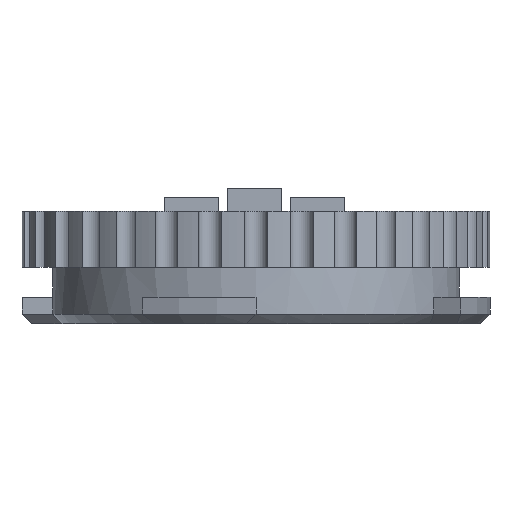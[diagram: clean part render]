
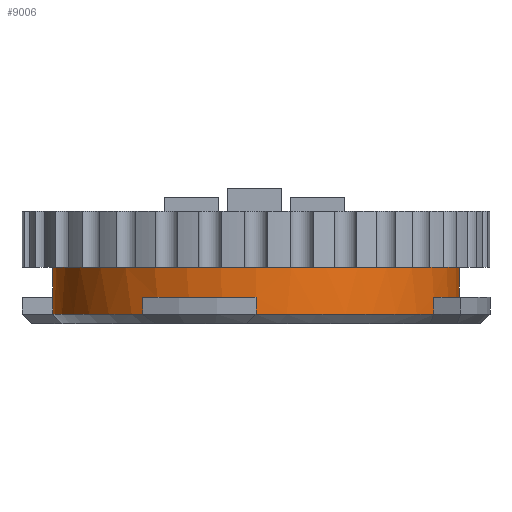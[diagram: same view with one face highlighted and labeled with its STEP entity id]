
A CAD part, front view. The second image highlights one B-rep face of the part: STEP entity #9006.
In plain terms, the highlighted cylindrical face has radius 13.787 mm (diameter 27.575 mm), a partial arc.
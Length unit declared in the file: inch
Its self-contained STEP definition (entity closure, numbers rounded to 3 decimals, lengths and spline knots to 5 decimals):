
#141 = EDGE_LOOP ( 'NONE', ( #9141, #763, #3634, #7107, #8365, #8469, #3518, #1365, #10371, #2251, #10949 ) ) ;
#189 = VECTOR ( 'NONE', #6156, 39.37008 ) ;
#298 = DIRECTION ( 'NONE',  ( 0., 0., 1. ) ) ;
#655 = LINE ( 'NONE', #5146, #10952 ) ;
#664 = DIRECTION ( 'NONE',  ( 1., 0., 0. ) ) ;
#696 = CARTESIAN_POINT ( 'NONE',  ( 0., 0., 0.02461 ) ) ;
#763 = ORIENTED_EDGE ( 'NONE', *, *, #4213, .F. ) ;
#806 = LINE ( 'NONE', #2953, #6941 ) ;
#832 = AXIS2_PLACEMENT_3D ( 'NONE', #9431, #8624, #664 ) ;
#866 = CARTESIAN_POINT ( 'NONE',  ( 0., -0.54281, 0.02461 ) ) ;
#1086 = DIRECTION ( 'NONE',  ( 0., 0., 1. ) ) ;
#1169 = CARTESIAN_POINT ( 'NONE',  ( 0.54281, 0., 0.15 ) ) ;
#1365 = ORIENTED_EDGE ( 'NONE', *, *, #7004, .T. ) ;
#1416 = DIRECTION ( 'NONE',  ( 1., 0., 0. ) ) ;
#1439 = CARTESIAN_POINT ( 'NONE',  ( 0., 0., 0.02461 ) ) ;
#1851 = VERTEX_POINT ( 'NONE', #9641 ) ;
#1888 = EDGE_CURVE ( 'NONE', #9745, #4321, #6204, .T. ) ;
#2251 = ORIENTED_EDGE ( 'NONE', *, *, #4976, .T. ) ;
#2330 = VERTEX_POINT ( 'NONE', #10304 ) ;
#2586 = CARTESIAN_POINT ( 'NONE',  ( 0., -0.54281, 0.15 ) ) ;
#2602 = DIRECTION ( 'NONE',  ( 0., 0., 1. ) ) ;
#2778 = CARTESIAN_POINT ( 'NONE',  ( -0.54281, 0., 0.07 ) ) ;
#2848 = DIRECTION ( 'NONE',  ( 0., 0., -1. ) ) ;
#2953 = CARTESIAN_POINT ( 'NONE',  ( -0.54281, 0., 0.15 ) ) ;
#2986 = EDGE_CURVE ( 'NONE', #6520, #3218, #8915, .T. ) ;
#3113 = EDGE_CURVE ( 'NONE', #11128, #8111, #8651, .T. ) ;
#3218 = VERTEX_POINT ( 'NONE', #11269 ) ;
#3281 = EDGE_CURVE ( 'NONE', #3218, #9745, #4130, .T. ) ;
#3293 = AXIS2_PLACEMENT_3D ( 'NONE', #7171, #298, #8107 ) ;
#3299 = CARTESIAN_POINT ( 'NONE',  ( 0.47476, -0.26316, 0.02461 ) ) ;
#3492 = VECTOR ( 'NONE', #2848, 39.37008 ) ;
#3518 = ORIENTED_EDGE ( 'NONE', *, *, #1888, .T. ) ;
#3634 = ORIENTED_EDGE ( 'NONE', *, *, #11001, .T. ) ;
#3752 = LINE ( 'NONE', #2586, #189 ) ;
#4087 = DIRECTION ( 'NONE',  ( 1., 0., 0. ) ) ;
#4117 = AXIS2_PLACEMENT_3D ( 'NONE', #9459, #7789, #7860 ) ;
#4130 = LINE ( 'NONE', #8966, #7940 ) ;
#4213 = EDGE_CURVE ( 'NONE', #1851, #10253, #10690, .T. ) ;
#4321 = VERTEX_POINT ( 'NONE', #9734 ) ;
#4491 = VECTOR ( 'NONE', #6603, 39.37008 ) ;
#4728 = LINE ( 'NONE', #1169, #3492 ) ;
#4976 = EDGE_CURVE ( 'NONE', #8111, #2330, #655, .T. ) ;
#5055 = VERTEX_POINT ( 'NONE', #2778 ) ;
#5146 = CARTESIAN_POINT ( 'NONE',  ( 0.47476, -0.26316, 0.15 ) ) ;
#5902 = DIRECTION ( 'NONE',  ( 0., 0., 1. ) ) ;
#6156 = DIRECTION ( 'NONE',  ( 0., 0., -1. ) ) ;
#6204 = CIRCLE ( 'NONE', #3293, 0.54281 ) ;
#6321 = FACE_OUTER_BOUND ( 'NONE', #141, .T. ) ;
#6477 = DIRECTION ( 'NONE',  ( 0., 0., -1. ) ) ;
#6520 = VERTEX_POINT ( 'NONE', #7871 ) ;
#6603 = DIRECTION ( 'NONE',  ( 0., 0., -1. ) ) ;
#6847 = DIRECTION ( 'NONE',  ( 1., 0., 0. ) ) ;
#6941 = VECTOR ( 'NONE', #6477, 39.37008 ) ;
#7004 = EDGE_CURVE ( 'NONE', #4321, #11128, #3752, .T. ) ;
#7107 = ORIENTED_EDGE ( 'NONE', *, *, #11328, .T. ) ;
#7136 = CYLINDRICAL_SURFACE ( 'NONE', #4117, 0.54281 ) ;
#7171 = CARTESIAN_POINT ( 'NONE',  ( 0., 0., 0.07 ) ) ;
#7276 = EDGE_CURVE ( 'NONE', #10253, #7650, #4728, .T. ) ;
#7650 = VERTEX_POINT ( 'NONE', #10517 ) ;
#7734 = DIRECTION ( 'NONE',  ( 0., 0., 1. ) ) ;
#7789 = DIRECTION ( 'NONE',  ( 0., 0., -1. ) ) ;
#7860 = DIRECTION ( 'NONE',  ( -1., 0., 0. ) ) ;
#7871 = CARTESIAN_POINT ( 'NONE',  ( -0.54281, 0., 0.02461 ) ) ;
#7940 = VECTOR ( 'NONE', #1086, 39.37008 ) ;
#8107 = DIRECTION ( 'NONE',  ( 0., -1., 0. ) ) ;
#8111 = VERTEX_POINT ( 'NONE', #3299 ) ;
#8365 = ORIENTED_EDGE ( 'NONE', *, *, #2986, .T. ) ;
#8469 = ORIENTED_EDGE ( 'NONE', *, *, #3281, .T. ) ;
#8619 = AXIS2_PLACEMENT_3D ( 'NONE', #8639, #7734, #6847 ) ;
#8624 = DIRECTION ( 'NONE',  ( 0., 0., 1. ) ) ;
#8639 = CARTESIAN_POINT ( 'NONE',  ( 0., 0., 0.15 ) ) ;
#8651 = CIRCLE ( 'NONE', #11045, 0.54281 ) ;
#8693 = CARTESIAN_POINT ( 'NONE',  ( 0.54281, 0., 0.15 ) ) ;
#8915 = CIRCLE ( 'NONE', #10442, 0.54281 ) ;
#8966 = CARTESIAN_POINT ( 'NONE',  ( -0.26316, -0.47476, 0.15 ) ) ;
#9006 = ADVANCED_FACE ( 'NONE', ( #6321 ), #7136, .T. ) ;
#9141 = ORIENTED_EDGE ( 'NONE', *, *, #7276, .F. ) ;
#9333 = DIRECTION ( 'NONE',  ( 0., 0., 1. ) ) ;
#9431 = CARTESIAN_POINT ( 'NONE',  ( 0., 0., 0.07 ) ) ;
#9459 = CARTESIAN_POINT ( 'NONE',  ( 0., 0., 0.15 ) ) ;
#9641 = CARTESIAN_POINT ( 'NONE',  ( -0.54281, 0., 0.15 ) ) ;
#9734 = CARTESIAN_POINT ( 'NONE',  ( 0., -0.54281, 0.07 ) ) ;
#9745 = VERTEX_POINT ( 'NONE', #10740 ) ;
#10101 = EDGE_CURVE ( 'NONE', #2330, #7650, #10848, .T. ) ;
#10253 = VERTEX_POINT ( 'NONE', #8693 ) ;
#10304 = CARTESIAN_POINT ( 'NONE',  ( 0.47476, -0.26316, 0.07 ) ) ;
#10371 = ORIENTED_EDGE ( 'NONE', *, *, #3113, .T. ) ;
#10442 = AXIS2_PLACEMENT_3D ( 'NONE', #696, #5902, #1416 ) ;
#10517 = CARTESIAN_POINT ( 'NONE',  ( 0.54281, 0., 0.07 ) ) ;
#10690 = CIRCLE ( 'NONE', #8619, 0.54281 ) ;
#10740 = CARTESIAN_POINT ( 'NONE',  ( -0.26316, -0.47476, 0.07 ) ) ;
#10848 = CIRCLE ( 'NONE', #832, 0.54281 ) ;
#10949 = ORIENTED_EDGE ( 'NONE', *, *, #10101, .T. ) ;
#10952 = VECTOR ( 'NONE', #2602, 39.37008 ) ;
#11001 = EDGE_CURVE ( 'NONE', #1851, #5055, #11386, .T. ) ;
#11045 = AXIS2_PLACEMENT_3D ( 'NONE', #1439, #9333, #4087 ) ;
#11123 = CARTESIAN_POINT ( 'NONE',  ( -0.54281, 0., 0.15 ) ) ;
#11128 = VERTEX_POINT ( 'NONE', #866 ) ;
#11269 = CARTESIAN_POINT ( 'NONE',  ( -0.26316, -0.47476, 0.02461 ) ) ;
#11328 = EDGE_CURVE ( 'NONE', #5055, #6520, #806, .T. ) ;
#11386 = LINE ( 'NONE', #11123, #4491 ) ;
